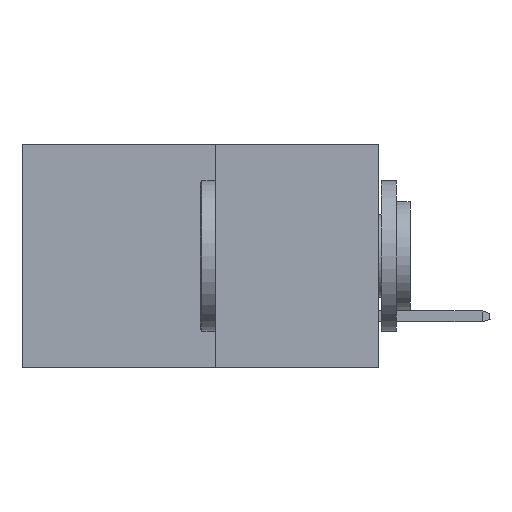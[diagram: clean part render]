
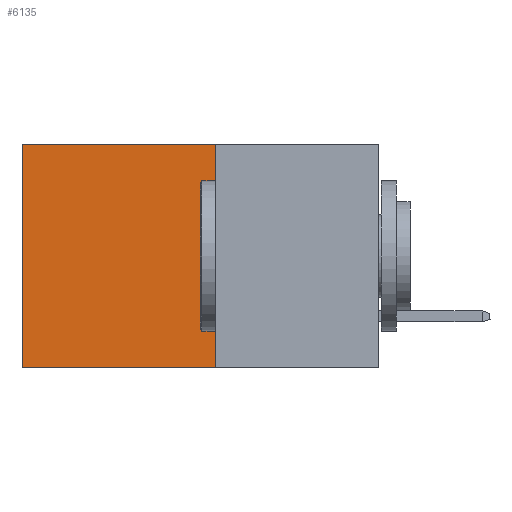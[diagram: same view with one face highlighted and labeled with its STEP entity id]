
A CAD part, left-side view. The second image highlights one B-rep face of the part: STEP entity #6135.
In plain terms, the highlighted planar face has unit normal (-1, 0, 0).
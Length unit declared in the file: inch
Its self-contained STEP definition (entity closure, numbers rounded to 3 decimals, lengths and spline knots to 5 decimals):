
#2341 = EDGE_CURVE ( 'NONE', #3287, #24543, #23796, .T. ) ;
#2623 = ORIENTED_EDGE ( 'NONE', *, *, #21607, .F. ) ;
#2683 = EDGE_LOOP ( 'NONE', ( #15881, #2623, #14054, #10853 ) ) ;
#3287 = VERTEX_POINT ( 'NONE', #10242 ) ;
#4249 = CARTESIAN_POINT ( 'NONE',  ( 0.277, 0.27, -0.37 ) ) ;
#4286 = CARTESIAN_POINT ( 'NONE',  ( 0.277, 0.27, -0.37 ) ) ;
#5241 = CARTESIAN_POINT ( 'NONE',  ( 0.277, 0.27, -0.37 ) ) ;
#5689 = VECTOR ( 'NONE', #9841, 39.37008 ) ;
#6135 = ADVANCED_FACE ( 'NONE', ( #8104 ), #11055, .F. ) ;
#6679 = DIRECTION ( 'NONE',  ( 0., 1., 0. ) ) ;
#7002 = VERTEX_POINT ( 'NONE', #19144 ) ;
#8104 = FACE_OUTER_BOUND ( 'NONE', #2683, .T. ) ;
#9352 = VECTOR ( 'NONE', #6679, 39.37008 ) ;
#9841 = DIRECTION ( 'NONE',  ( 0., 0., -1. ) ) ;
#10242 = CARTESIAN_POINT ( 'NONE',  ( 0.277, 0.27, 0. ) ) ;
#10853 = ORIENTED_EDGE ( 'NONE', *, *, #29614, .T. ) ;
#10952 = DIRECTION ( 'NONE',  ( 0., 0., -1. ) ) ;
#10991 = DIRECTION ( 'NONE',  ( 1., 0., 0. ) ) ;
#11055 = PLANE ( 'NONE',  #16636 ) ;
#11156 = CARTESIAN_POINT ( 'NONE',  ( 0.277, 0.27, -0.37 ) ) ;
#13887 = EDGE_CURVE ( 'NONE', #7002, #30027, #26942, .T. ) ;
#14054 = ORIENTED_EDGE ( 'NONE', *, *, #2341, .F. ) ;
#15632 = LINE ( 'NONE', #26297, #27323 ) ;
#15692 = LINE ( 'NONE', #4286, #9352 ) ;
#15881 = ORIENTED_EDGE ( 'NONE', *, *, #13887, .T. ) ;
#16421 = CARTESIAN_POINT ( 'NONE',  ( 0.277, 0.59, -0.37 ) ) ;
#16636 = AXIS2_PLACEMENT_3D ( 'NONE', #11156, #10991, #10952 ) ;
#18770 = DIRECTION ( 'NONE',  ( 0., 0., -1. ) ) ;
#19144 = CARTESIAN_POINT ( 'NONE',  ( 0.277, 0.59, 0. ) ) ;
#21607 = EDGE_CURVE ( 'NONE', #24543, #30027, #15692, .T. ) ;
#23796 = LINE ( 'NONE', #5241, #5689 ) ;
#24543 = VERTEX_POINT ( 'NONE', #4249 ) ;
#25248 = CARTESIAN_POINT ( 'NONE',  ( 0.277, 0.59, -0.37 ) ) ;
#26297 = CARTESIAN_POINT ( 'NONE',  ( 0.277, 0.27, 0. ) ) ;
#26942 = LINE ( 'NONE', #16421, #30181 ) ;
#27323 = VECTOR ( 'NONE', #28606, 39.37008 ) ;
#28606 = DIRECTION ( 'NONE',  ( 0., 1., 0. ) ) ;
#29614 = EDGE_CURVE ( 'NONE', #3287, #7002, #15632, .T. ) ;
#30027 = VERTEX_POINT ( 'NONE', #25248 ) ;
#30181 = VECTOR ( 'NONE', #18770, 39.37008 ) ;
